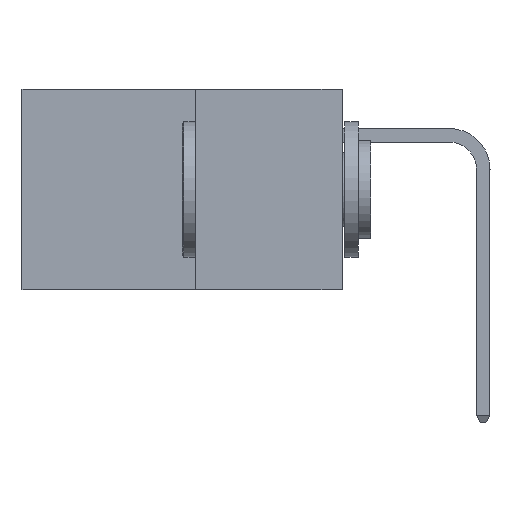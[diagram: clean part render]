
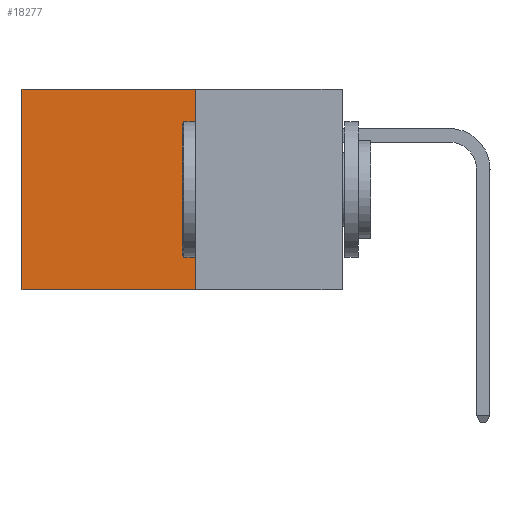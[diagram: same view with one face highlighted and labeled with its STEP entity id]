
A CAD part, left-side view. The second image highlights one B-rep face of the part: STEP entity #18277.
In plain terms, the highlighted planar face has unit normal (-1, 0, 0).
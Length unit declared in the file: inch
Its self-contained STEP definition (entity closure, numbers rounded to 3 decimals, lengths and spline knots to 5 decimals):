
#72 = CARTESIAN_POINT ( 'NONE',  ( 0.277, 0.27, 0. ) ) ;
#75 = CARTESIAN_POINT ( 'NONE',  ( 0.277, 0.27, -0.37 ) ) ;
#793 = EDGE_CURVE ( 'NONE', #13405, #9887, #11314, .T. ) ;
#2676 = ORIENTED_EDGE ( 'NONE', *, *, #6559, .F. ) ;
#4200 = VERTEX_POINT ( 'NONE', #12568 ) ;
#4384 = ORIENTED_EDGE ( 'NONE', *, *, #17508, .F. ) ;
#4412 = VECTOR ( 'NONE', #8275, 39.37008 ) ;
#4929 = EDGE_LOOP ( 'NONE', ( #8875, #2676, #4384, #19517 ) ) ;
#5629 = AXIS2_PLACEMENT_3D ( 'NONE', #10313, #22262, #12028 ) ;
#6276 = LINE ( 'NONE', #7381, #15013 ) ;
#6492 = CARTESIAN_POINT ( 'NONE',  ( 0.277, 0.27, -0.37 ) ) ;
#6559 = EDGE_CURVE ( 'NONE', #16619, #4200, #8298, .T. ) ;
#7381 = CARTESIAN_POINT ( 'NONE',  ( 0.277, 0.59, -0.37 ) ) ;
#8275 = DIRECTION ( 'NONE',  ( 0., 0., -1. ) ) ;
#8298 = LINE ( 'NONE', #75, #9410 ) ;
#8472 = CARTESIAN_POINT ( 'NONE',  ( 0.277, 0.27, -0.37 ) ) ;
#8818 = CARTESIAN_POINT ( 'NONE',  ( 0.277, 0.59, 0. ) ) ;
#8875 = ORIENTED_EDGE ( 'NONE', *, *, #18533, .T. ) ;
#9410 = VECTOR ( 'NONE', #19050, 39.37008 ) ;
#9887 = VERTEX_POINT ( 'NONE', #8818 ) ;
#10313 = CARTESIAN_POINT ( 'NONE',  ( 0.277, 0.27, -0.37 ) ) ;
#11314 = LINE ( 'NONE', #17180, #19435 ) ;
#12028 = DIRECTION ( 'NONE',  ( 0., 0., -1. ) ) ;
#12568 = CARTESIAN_POINT ( 'NONE',  ( 0.277, 0.59, -0.37 ) ) ;
#13405 = VERTEX_POINT ( 'NONE', #72 ) ;
#15013 = VECTOR ( 'NONE', #21182, 39.37008 ) ;
#16619 = VERTEX_POINT ( 'NONE', #8472 ) ;
#17180 = CARTESIAN_POINT ( 'NONE',  ( 0.277, 0.27, 0. ) ) ;
#17234 = PLANE ( 'NONE',  #5629 ) ;
#17508 = EDGE_CURVE ( 'NONE', #13405, #16619, #18349, .T. ) ;
#18277 = ADVANCED_FACE ( 'NONE', ( #20893 ), #17234, .F. ) ;
#18349 = LINE ( 'NONE', #6492, #4412 ) ;
#18533 = EDGE_CURVE ( 'NONE', #9887, #4200, #6276, .T. ) ;
#18689 = DIRECTION ( 'NONE',  ( 0., 1., 0. ) ) ;
#19050 = DIRECTION ( 'NONE',  ( 0., 1., 0. ) ) ;
#19435 = VECTOR ( 'NONE', #18689, 39.37008 ) ;
#19517 = ORIENTED_EDGE ( 'NONE', *, *, #793, .T. ) ;
#20893 = FACE_OUTER_BOUND ( 'NONE', #4929, .T. ) ;
#21182 = DIRECTION ( 'NONE',  ( 0., 0., -1. ) ) ;
#22262 = DIRECTION ( 'NONE',  ( 1., 0., 0. ) ) ;
